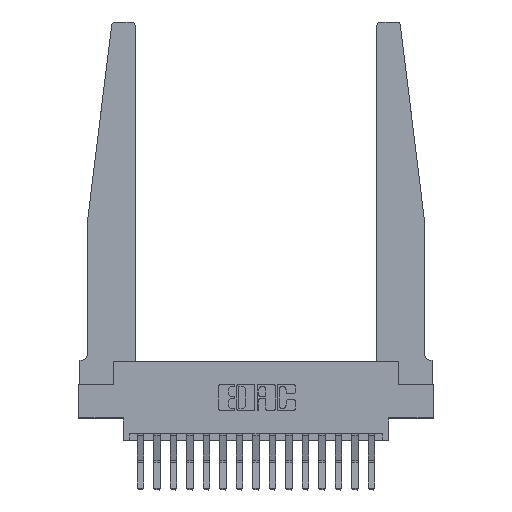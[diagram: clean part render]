
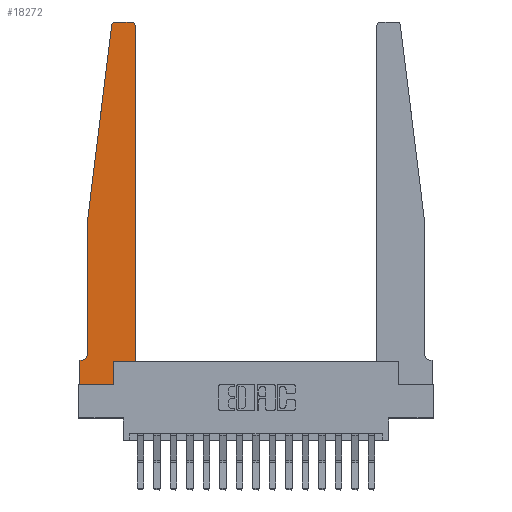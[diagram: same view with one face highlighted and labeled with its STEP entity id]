
A CAD part, top view. The second image highlights one B-rep face of the part: STEP entity #18272.
In plain terms, the highlighted planar face has unit normal (0, 0, 1).
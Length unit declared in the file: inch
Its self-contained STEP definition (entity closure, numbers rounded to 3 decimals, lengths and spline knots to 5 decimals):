
#285 = EDGE_CURVE ( 'NONE', #13606, #5848, #15020, .T. ) ;
#323 = CIRCLE ( 'NONE', #8825, 0.03 ) ;
#329 = DIRECTION ( 'NONE',  ( 0., 0., -1. ) ) ;
#609 = ORIENTED_EDGE ( 'NONE', *, *, #12958, .T. ) ;
#921 = VECTOR ( 'NONE', #18159, 39.37008 ) ;
#1136 = DIRECTION ( 'NONE',  ( 1., 0., 0. ) ) ;
#1297 = DIRECTION ( 'NONE',  ( 1., 0., 0. ) ) ;
#1953 = EDGE_CURVE ( 'NONE', #4356, #4629, #14633, .T. ) ;
#2006 = CIRCLE ( 'NONE', #9304, 0.05 ) ;
#2372 = ORIENTED_EDGE ( 'NONE', *, *, #4911, .T. ) ;
#2452 = PLANE ( 'NONE',  #8357 ) ;
#2476 = LINE ( 'NONE', #9537, #11177 ) ;
#2575 = LINE ( 'NONE', #15368, #12649 ) ;
#2754 = CARTESIAN_POINT ( 'NONE',  ( 0.24675, 2.72367, 0.37 ) ) ;
#2790 = CARTESIAN_POINT ( 'NONE',  ( 0.2605, 0.18, 0.37 ) ) ;
#2999 = CARTESIAN_POINT ( 'NONE',  ( 0.27653, 2.75, 0.37 ) ) ;
#3082 = CARTESIAN_POINT ( 'NONE',  ( 0.2605, 0.18, 0.37 ) ) ;
#3119 = DIRECTION ( 'NONE',  ( 1., 0., 0. ) ) ;
#3146 = CARTESIAN_POINT ( 'NONE',  ( 0.015, 0.1875, 0.37 ) ) ;
#3251 = ORIENTED_EDGE ( 'NONE', *, *, #285, .T. ) ;
#3429 = DIRECTION ( 'NONE',  ( 1., 0., 0. ) ) ;
#3457 = CARTESIAN_POINT ( 'NONE',  ( 0.2605, 0., 0.37 ) ) ;
#3783 = VECTOR ( 'NONE', #3119, 39.37008 ) ;
#3847 = EDGE_CURVE ( 'NONE', #5393, #4356, #18491, .T. ) ;
#3876 = FACE_OUTER_BOUND ( 'NONE', #4379, .T. ) ;
#3922 = EDGE_CURVE ( 'NONE', #4629, #6891, #17808, .T. ) ;
#4316 = VERTEX_POINT ( 'NONE', #2999 ) ;
#4356 = VERTEX_POINT ( 'NONE', #3457 ) ;
#4379 = EDGE_LOOP ( 'NONE', ( #10120, #10406, #14085, #15981, #2372, #3251, #14648, #18844, #14544, #10547, #609, #6420 ) ) ;
#4629 = VERTEX_POINT ( 'NONE', #2790 ) ;
#4682 = CARTESIAN_POINT ( 'NONE',  ( 0.065, 0.2375, 0.37 ) ) ;
#4875 = CARTESIAN_POINT ( 'NONE',  ( 0.065, 1.25, 0.37 ) ) ;
#4911 = EDGE_CURVE ( 'NONE', #17540, #13606, #2006, .T. ) ;
#5000 = EDGE_CURVE ( 'NONE', #5848, #5393, #2575, .T. ) ;
#5393 = VERTEX_POINT ( 'NONE', #11394 ) ;
#5650 = CARTESIAN_POINT ( 'NONE',  ( 0.425, 0.18, 0.37 ) ) ;
#5848 = VERTEX_POINT ( 'NONE', #18835 ) ;
#6069 = CARTESIAN_POINT ( 'NONE',  ( 0.425, 0.18, 0.37 ) ) ;
#6392 = CARTESIAN_POINT ( 'NONE',  ( 0.395, 2.72, 0.37 ) ) ;
#6420 = ORIENTED_EDGE ( 'NONE', *, *, #9222, .T. ) ;
#6689 = EDGE_CURVE ( 'NONE', #11722, #17540, #2476, .T. ) ;
#6704 = VECTOR ( 'NONE', #17299, 39.37008 ) ;
#6779 = DIRECTION ( 'NONE',  ( 0., -1., 0. ) ) ;
#6891 = VERTEX_POINT ( 'NONE', #17714 ) ;
#7393 = VECTOR ( 'NONE', #18358, 39.37008 ) ;
#8357 = AXIS2_PLACEMENT_3D ( 'NONE', #12945, #18676, #11320 ) ;
#8540 = CARTESIAN_POINT ( 'NONE',  ( 0.27653, 2.72, 0.37 ) ) ;
#8637 = VERTEX_POINT ( 'NONE', #14449 ) ;
#8825 = AXIS2_PLACEMENT_3D ( 'NONE', #8540, #14361, #1297 ) ;
#9222 = EDGE_CURVE ( 'NONE', #8637, #15814, #10631, .T. ) ;
#9304 = AXIS2_PLACEMENT_3D ( 'NONE', #13662, #329, #17763 ) ;
#9537 = CARTESIAN_POINT ( 'NONE',  ( 0.065, 1.25, 0.37 ) ) ;
#9918 = EDGE_CURVE ( 'NONE', #4316, #14003, #323, .T. ) ;
#9958 = VECTOR ( 'NONE', #10422, 39.37008 ) ;
#10033 = AXIS2_PLACEMENT_3D ( 'NONE', #6392, #18036, #3429 ) ;
#10120 = ORIENTED_EDGE ( 'NONE', *, *, #15862, .T. ) ;
#10127 = EDGE_CURVE ( 'NONE', #14003, #11722, #15293, .T. ) ;
#10406 = ORIENTED_EDGE ( 'NONE', *, *, #9918, .T. ) ;
#10419 = LINE ( 'NONE', #5650, #6704 ) ;
#10422 = DIRECTION ( 'NONE',  ( 0., 1., 0. ) ) ;
#10547 = ORIENTED_EDGE ( 'NONE', *, *, #3922, .T. ) ;
#10631 = CIRCLE ( 'NONE', #10033, 0.03 ) ;
#11177 = VECTOR ( 'NONE', #14030, 39.37008 ) ;
#11320 = DIRECTION ( 'NONE',  ( 1., 0., 0. ) ) ;
#11324 = CARTESIAN_POINT ( 'NONE',  ( 0., 0., 0.37 ) ) ;
#11394 = CARTESIAN_POINT ( 'NONE',  ( 0., 0., 0.37 ) ) ;
#11714 = VECTOR ( 'NONE', #1136, 39.37008 ) ;
#11722 = VERTEX_POINT ( 'NONE', #4875 ) ;
#11869 = CARTESIAN_POINT ( 'NONE',  ( 0.065, 0.1875, 0.37 ) ) ;
#12527 = CARTESIAN_POINT ( 'NONE',  ( 0.25, 2.75, 0.37 ) ) ;
#12649 = VECTOR ( 'NONE', #6779, 39.37008 ) ;
#12945 = CARTESIAN_POINT ( 'NONE',  ( 0., 0.1875, 0.37 ) ) ;
#12958 = EDGE_CURVE ( 'NONE', #6891, #8637, #10419, .T. ) ;
#13606 = VERTEX_POINT ( 'NONE', #3146 ) ;
#13662 = CARTESIAN_POINT ( 'NONE',  ( 0.015, 0.2375, 0.37 ) ) ;
#13863 = CARTESIAN_POINT ( 'NONE',  ( 0.065, 1.25, 0.37 ) ) ;
#13981 = LINE ( 'NONE', #12527, #7393 ) ;
#14003 = VERTEX_POINT ( 'NONE', #2754 ) ;
#14030 = DIRECTION ( 'NONE',  ( 0., -1., 0. ) ) ;
#14085 = ORIENTED_EDGE ( 'NONE', *, *, #10127, .T. ) ;
#14361 = DIRECTION ( 'NONE',  ( 0., 0., 1. ) ) ;
#14449 = CARTESIAN_POINT ( 'NONE',  ( 0.425, 2.72, 0.37 ) ) ;
#14544 = ORIENTED_EDGE ( 'NONE', *, *, #1953, .T. ) ;
#14633 = LINE ( 'NONE', #3082, #9958 ) ;
#14648 = ORIENTED_EDGE ( 'NONE', *, *, #5000, .T. ) ;
#15020 = LINE ( 'NONE', #11869, #16785 ) ;
#15293 = LINE ( 'NONE', #13863, #921 ) ;
#15368 = CARTESIAN_POINT ( 'NONE',  ( 0., 0., 0.37 ) ) ;
#15814 = VERTEX_POINT ( 'NONE', #18460 ) ;
#15862 = EDGE_CURVE ( 'NONE', #15814, #4316, #13981, .T. ) ;
#15981 = ORIENTED_EDGE ( 'NONE', *, *, #6689, .T. ) ;
#16084 = DIRECTION ( 'NONE',  ( -1., 0., 0. ) ) ;
#16785 = VECTOR ( 'NONE', #16084, 39.37008 ) ;
#17299 = DIRECTION ( 'NONE',  ( 0., 1., 0. ) ) ;
#17540 = VERTEX_POINT ( 'NONE', #4682 ) ;
#17714 = CARTESIAN_POINT ( 'NONE',  ( 0.425, 0.18, 0.37 ) ) ;
#17763 = DIRECTION ( 'NONE',  ( -1., 0., 0. ) ) ;
#17808 = LINE ( 'NONE', #6069, #3783 ) ;
#18036 = DIRECTION ( 'NONE',  ( 0., 0., 1. ) ) ;
#18159 = DIRECTION ( 'NONE',  ( -0.122, -0.992, 0. ) ) ;
#18272 = ADVANCED_FACE ( 'NONE', ( #3876 ), #2452, .T. ) ;
#18358 = DIRECTION ( 'NONE',  ( -1., 0., 0. ) ) ;
#18460 = CARTESIAN_POINT ( 'NONE',  ( 0.395, 2.75, 0.37 ) ) ;
#18491 = LINE ( 'NONE', #11324, #11714 ) ;
#18676 = DIRECTION ( 'NONE',  ( 0., 0., 1. ) ) ;
#18835 = CARTESIAN_POINT ( 'NONE',  ( 0., 0.1875, 0.37 ) ) ;
#18844 = ORIENTED_EDGE ( 'NONE', *, *, #3847, .T. ) ;
